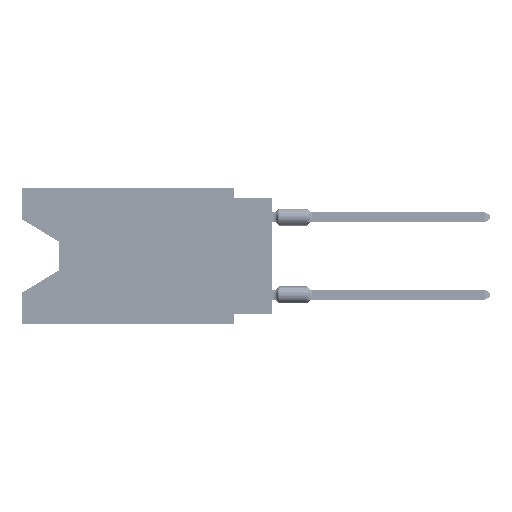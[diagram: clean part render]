
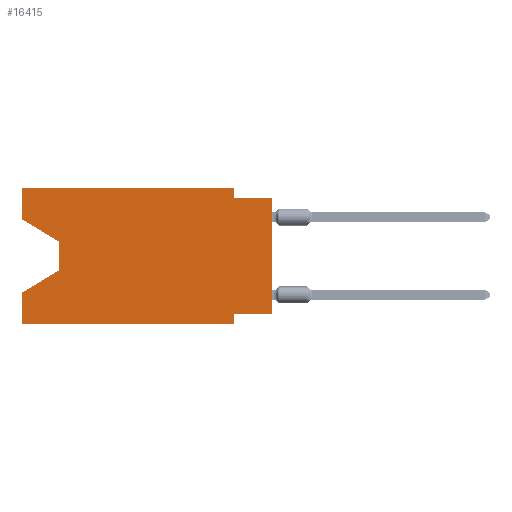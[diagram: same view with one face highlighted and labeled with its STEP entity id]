
A CAD part, left-side view. The second image highlights one B-rep face of the part: STEP entity #16415.
In plain terms, the highlighted planar face has unit normal (-1, 0, 0).
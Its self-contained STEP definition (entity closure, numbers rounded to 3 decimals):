
#1269 = CARTESIAN_POINT ( 'NONE',  ( 0., 16.383, -8.89 ) ) ;
#1587 = EDGE_CURVE ( 'NONE', #6960, #22802, #23411, .T. ) ;
#3395 = LINE ( 'NONE', #25790, #60749 ) ;
#4560 = CARTESIAN_POINT ( 'NONE',  ( 0., 2.54, -8.89 ) ) ;
#5040 = ORIENTED_EDGE ( 'NONE', *, *, #42470, .F. ) ;
#5304 = LINE ( 'NONE', #26661, #59054 ) ;
#5363 = VERTEX_POINT ( 'NONE', #26336 ) ;
#5505 = ORIENTED_EDGE ( 'NONE', *, *, #48959, .F. ) ;
#5546 = CARTESIAN_POINT ( 'NONE',  ( 0., 0., 0. ) ) ;
#6960 = VERTEX_POINT ( 'NONE', #1269 ) ;
#7602 = AXIS2_PLACEMENT_3D ( 'NONE', #7885, #61423, #66694 ) ;
#7688 = VECTOR ( 'NONE', #32486, 1000. ) ;
#7855 = LINE ( 'NONE', #28180, #68456 ) ;
#7885 = CARTESIAN_POINT ( 'NONE',  ( 0., 16.383, 0. ) ) ;
#8560 = CARTESIAN_POINT ( 'NONE',  ( 0., 2.54, -8.255 ) ) ;
#9591 = EDGE_LOOP ( 'NONE', ( #46476, #57164, #53756, #53564, #39280, #28319, #55204, #15363, #5040, #67290, #21065, #5505 ) ) ;
#10464 = LINE ( 'NONE', #5546, #7688 ) ;
#10832 = CARTESIAN_POINT ( 'NONE',  ( 0., 2.54, 0. ) ) ;
#10841 = DIRECTION ( 'NONE',  ( 0., -0.855, -0.519 ) ) ;
#11612 = EDGE_CURVE ( 'NONE', #33319, #58031, #31145, .T. ) ;
#14679 = LINE ( 'NONE', #57016, #62385 ) ;
#15363 = ORIENTED_EDGE ( 'NONE', *, *, #22031, .T. ) ;
#15651 = CARTESIAN_POINT ( 'NONE',  ( 0., 16.383, -2.038 ) ) ;
#16252 = CARTESIAN_POINT ( 'NONE',  ( 0., 2.54, 0. ) ) ;
#16415 = ADVANCED_FACE ( 'NONE', ( #28567 ), #49915, .F. ) ;
#17487 = CARTESIAN_POINT ( 'NONE',  ( 0., 16.383, 0. ) ) ;
#18765 = EDGE_CURVE ( 'NONE', #24069, #67063, #3395, .T. ) ;
#21065 = ORIENTED_EDGE ( 'NONE', *, *, #18765, .F. ) ;
#21160 = LINE ( 'NONE', #58602, #39356 ) ;
#21389 = LINE ( 'NONE', #64080, #65411 ) ;
#21678 = DIRECTION ( 'NONE',  ( 0., 0., -1. ) ) ;
#21782 = DIRECTION ( 'NONE',  ( 0., 0., 1. ) ) ;
#22031 = EDGE_CURVE ( 'NONE', #55765, #31877, #10464, .T. ) ;
#22353 = LINE ( 'NONE', #10832, #38400 ) ;
#22802 = VERTEX_POINT ( 'NONE', #62363 ) ;
#22865 = VERTEX_POINT ( 'NONE', #43097 ) ;
#22924 = EDGE_CURVE ( 'NONE', #58031, #5363, #5304, .T. ) ;
#23411 = LINE ( 'NONE', #17487, #42454 ) ;
#24069 = VERTEX_POINT ( 'NONE', #64200 ) ;
#25790 = CARTESIAN_POINT ( 'NONE',  ( 0., 16.383, 0. ) ) ;
#25917 = DIRECTION ( 'NONE',  ( 0., 0., -1. ) ) ;
#26336 = CARTESIAN_POINT ( 'NONE',  ( 0., 13.97, -5.385 ) ) ;
#26661 = CARTESIAN_POINT ( 'NONE',  ( 0., 13.97, -3.505 ) ) ;
#26931 = CARTESIAN_POINT ( 'NONE',  ( 0., 16.383, -2.038 ) ) ;
#26978 = DIRECTION ( 'NONE',  ( 0., 1., 0. ) ) ;
#28180 = CARTESIAN_POINT ( 'NONE',  ( 0., 16.383, -8.89 ) ) ;
#28319 = ORIENTED_EDGE ( 'NONE', *, *, #54025, .F. ) ;
#28567 = FACE_OUTER_BOUND ( 'NONE', #9591, .T. ) ;
#31145 = LINE ( 'NONE', #26931, #53774 ) ;
#31509 = EDGE_CURVE ( 'NONE', #5363, #22802, #14679, .T. ) ;
#31877 = VERTEX_POINT ( 'NONE', #34551 ) ;
#32486 = DIRECTION ( 'NONE',  ( 0., 0., 1. ) ) ;
#32921 = EDGE_CURVE ( 'NONE', #67063, #22865, #22353, .T. ) ;
#33023 = DIRECTION ( 'NONE',  ( 0., 0., 1. ) ) ;
#33319 = VERTEX_POINT ( 'NONE', #15651 ) ;
#34551 = CARTESIAN_POINT ( 'NONE',  ( 0., 0., -0.635 ) ) ;
#35095 = VECTOR ( 'NONE', #25917, 1000. ) ;
#35119 = LINE ( 'NONE', #52256, #37200 ) ;
#37200 = VECTOR ( 'NONE', #46664, 1000. ) ;
#38400 = VECTOR ( 'NONE', #21678, 1000. ) ;
#39280 = ORIENTED_EDGE ( 'NONE', *, *, #47354, .T. ) ;
#39356 = VECTOR ( 'NONE', #33023, 1000. ) ;
#41612 = DIRECTION ( 'NONE',  ( 0., 0.855, -0.519 ) ) ;
#42454 = VECTOR ( 'NONE', #21782, 1000. ) ;
#42470 = EDGE_CURVE ( 'NONE', #22865, #31877, #35119, .T. ) ;
#43097 = CARTESIAN_POINT ( 'NONE',  ( 0., 2.54, -0.635 ) ) ;
#46476 = ORIENTED_EDGE ( 'NONE', *, *, #11612, .T. ) ;
#46664 = DIRECTION ( 'NONE',  ( 0., -1., 0. ) ) ;
#46837 = CARTESIAN_POINT ( 'NONE',  ( 0., 13.97, -3.505 ) ) ;
#47354 = EDGE_CURVE ( 'NONE', #6960, #65545, #7855, .T. ) ;
#47550 = CARTESIAN_POINT ( 'NONE',  ( 0., 0., -8.255 ) ) ;
#48001 = DIRECTION ( 'NONE',  ( 0., 0., -1. ) ) ;
#48959 = EDGE_CURVE ( 'NONE', #33319, #24069, #21160, .T. ) ;
#49915 = PLANE ( 'NONE',  #7602 ) ;
#51947 = EDGE_CURVE ( 'NONE', #55765, #64960, #21389, .T. ) ;
#52256 = CARTESIAN_POINT ( 'NONE',  ( 0., 0., -0.635 ) ) ;
#53564 = ORIENTED_EDGE ( 'NONE', *, *, #1587, .F. ) ;
#53756 = ORIENTED_EDGE ( 'NONE', *, *, #31509, .T. ) ;
#53774 = VECTOR ( 'NONE', #10841, 1000. ) ;
#54025 = EDGE_CURVE ( 'NONE', #64960, #65545, #57763, .T. ) ;
#55126 = DIRECTION ( 'NONE',  ( 0., -1., 0. ) ) ;
#55204 = ORIENTED_EDGE ( 'NONE', *, *, #51947, .F. ) ;
#55765 = VERTEX_POINT ( 'NONE', #47550 ) ;
#57016 = CARTESIAN_POINT ( 'NONE',  ( 0., 13.97, -5.385 ) ) ;
#57164 = ORIENTED_EDGE ( 'NONE', *, *, #22924, .T. ) ;
#57763 = LINE ( 'NONE', #4560, #35095 ) ;
#58031 = VERTEX_POINT ( 'NONE', #46837 ) ;
#58602 = CARTESIAN_POINT ( 'NONE',  ( 0., 16.383, 0. ) ) ;
#59054 = VECTOR ( 'NONE', #48001, 1000. ) ;
#60749 = VECTOR ( 'NONE', #62195, 1000. ) ;
#61423 = DIRECTION ( 'NONE',  ( 1., 0., 0. ) ) ;
#62195 = DIRECTION ( 'NONE',  ( 0., -1., 0. ) ) ;
#62363 = CARTESIAN_POINT ( 'NONE',  ( 0., 16.383, -6.852 ) ) ;
#62385 = VECTOR ( 'NONE', #41612, 1000. ) ;
#64080 = CARTESIAN_POINT ( 'NONE',  ( 0., 0., -8.255 ) ) ;
#64200 = CARTESIAN_POINT ( 'NONE',  ( 0., 16.383, 0. ) ) ;
#64960 = VERTEX_POINT ( 'NONE', #8560 ) ;
#65411 = VECTOR ( 'NONE', #26978, 1000. ) ;
#65545 = VERTEX_POINT ( 'NONE', #66720 ) ;
#66694 = DIRECTION ( 'NONE',  ( 0., 0., -1. ) ) ;
#66720 = CARTESIAN_POINT ( 'NONE',  ( 0., 2.54, -8.89 ) ) ;
#67063 = VERTEX_POINT ( 'NONE', #16252 ) ;
#67290 = ORIENTED_EDGE ( 'NONE', *, *, #32921, .F. ) ;
#68456 = VECTOR ( 'NONE', #55126, 1000. ) ;
